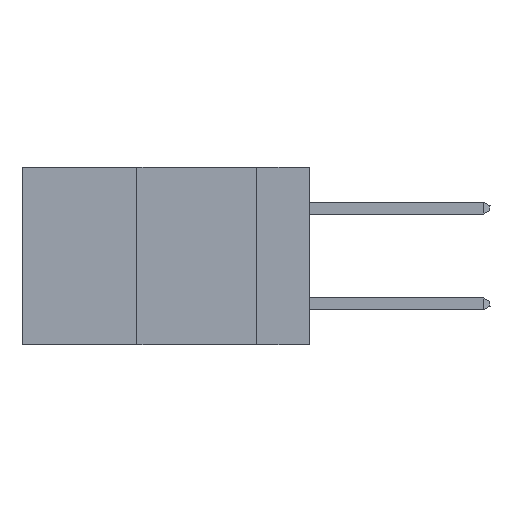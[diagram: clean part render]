
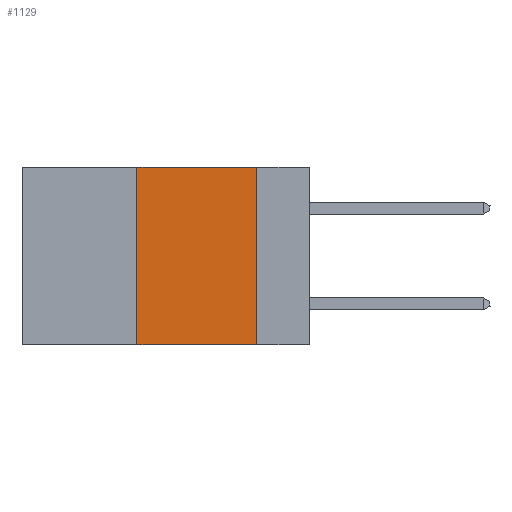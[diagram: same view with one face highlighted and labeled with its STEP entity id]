
A CAD part, left-side view. The second image highlights one B-rep face of the part: STEP entity #1129.
In plain terms, the highlighted planar face has unit normal (-1, 0, 0).
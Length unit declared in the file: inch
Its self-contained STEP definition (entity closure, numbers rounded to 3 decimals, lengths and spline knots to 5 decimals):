
#289 = CARTESIAN_POINT ( 'NONE',  ( 0., 0.36, -0.37 ) ) ;
#1038 = VECTOR ( 'NONE', #10147, 39.37008 ) ;
#1129 = ADVANCED_FACE ( 'NONE', ( #23190 ), #2697, .F. ) ;
#2697 = PLANE ( 'NONE',  #20289 ) ;
#3209 = CARTESIAN_POINT ( 'NONE',  ( 0., 0.11, -0.37 ) ) ;
#3436 = CARTESIAN_POINT ( 'NONE',  ( 0., 0.11, 0. ) ) ;
#4251 = EDGE_CURVE ( 'NONE', #9171, #17124, #19695, .T. ) ;
#4517 = CARTESIAN_POINT ( 'NONE',  ( 0., 0.6, 0. ) ) ;
#4626 = CARTESIAN_POINT ( 'NONE',  ( 0., 0.6, -0.37 ) ) ;
#7725 = EDGE_LOOP ( 'NONE', ( #18289, #10049, #22499, #21396 ) ) ;
#8353 = VERTEX_POINT ( 'NONE', #22710 ) ;
#8398 = LINE ( 'NONE', #12359, #1038 ) ;
#8725 = VERTEX_POINT ( 'NONE', #15606 ) ;
#9126 = LINE ( 'NONE', #3436, #23249 ) ;
#9155 = DIRECTION ( 'NONE',  ( 0., -1., 0. ) ) ;
#9171 = VERTEX_POINT ( 'NONE', #289 ) ;
#10049 = ORIENTED_EDGE ( 'NONE', *, *, #21187, .F. ) ;
#10147 = DIRECTION ( 'NONE',  ( 0., 0., 1. ) ) ;
#12359 = CARTESIAN_POINT ( 'NONE',  ( 0., 0.36, 0. ) ) ;
#13361 = CARTESIAN_POINT ( 'NONE',  ( 0., 0.6, 0. ) ) ;
#15606 = CARTESIAN_POINT ( 'NONE',  ( 0., 0.11, 0. ) ) ;
#15761 = EDGE_CURVE ( 'NONE', #8725, #17124, #9126, .T. ) ;
#16499 = EDGE_CURVE ( 'NONE', #9171, #8353, #8398, .T. ) ;
#17124 = VERTEX_POINT ( 'NONE', #3209 ) ;
#17509 = DIRECTION ( 'NONE',  ( 1., 0., 0. ) ) ;
#18289 = ORIENTED_EDGE ( 'NONE', *, *, #15761, .F. ) ;
#19695 = LINE ( 'NONE', #4626, #26062 ) ;
#20111 = VECTOR ( 'NONE', #9155, 39.37008 ) ;
#20289 = AXIS2_PLACEMENT_3D ( 'NONE', #4517, #17509, #21868 ) ;
#21187 = EDGE_CURVE ( 'NONE', #8353, #8725, #23143, .T. ) ;
#21396 = ORIENTED_EDGE ( 'NONE', *, *, #4251, .T. ) ;
#21796 = DIRECTION ( 'NONE',  ( 0., -1., 0. ) ) ;
#21868 = DIRECTION ( 'NONE',  ( 0., 0., -1. ) ) ;
#22499 = ORIENTED_EDGE ( 'NONE', *, *, #16499, .F. ) ;
#22710 = CARTESIAN_POINT ( 'NONE',  ( 0., 0.36, 0. ) ) ;
#22955 = DIRECTION ( 'NONE',  ( 0., 0., -1. ) ) ;
#23143 = LINE ( 'NONE', #13361, #20111 ) ;
#23190 = FACE_OUTER_BOUND ( 'NONE', #7725, .T. ) ;
#23249 = VECTOR ( 'NONE', #22955, 39.37008 ) ;
#26062 = VECTOR ( 'NONE', #21796, 39.37008 ) ;
